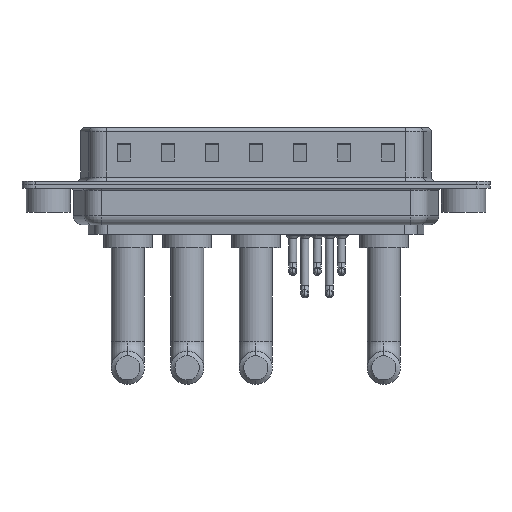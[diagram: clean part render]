
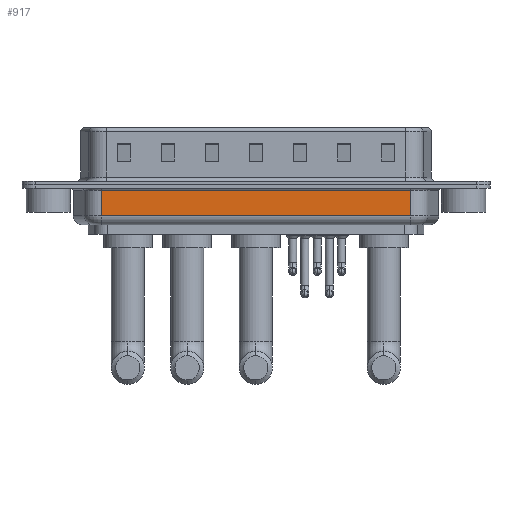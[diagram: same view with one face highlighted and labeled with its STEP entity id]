
A CAD part, front view. The second image highlights one B-rep face of the part: STEP entity #917.
In plain terms, the highlighted planar face has unit normal (0, -1, 0).
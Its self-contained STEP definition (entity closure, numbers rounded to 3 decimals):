
#821 = LINE ( 'NONE', #9465, #14283 ) ;
#917 = ADVANCED_FACE ( 'NONE', ( #13950 ), #20896, .F. ) ;
#1892 = DIRECTION ( 'NONE',  ( 0., 1., 0. ) ) ;
#2597 = CARTESIAN_POINT ( 'NONE',  ( 41.044, -5.35, -0.65 ) ) ;
#3189 = CARTESIAN_POINT ( 'NONE',  ( 6.006, -5.35, -0.65 ) ) ;
#3384 = EDGE_CURVE ( 'NONE', #19903, #16045, #821, .T. ) ;
#3623 = CARTESIAN_POINT ( 'NONE',  ( 6.006, -5.35, -0.65 ) ) ;
#4124 = DIRECTION ( 'NONE',  ( 1., 0., 0. ) ) ;
#4196 = EDGE_LOOP ( 'NONE', ( #12258, #13780, #5738, #14196 ) ) ;
#4897 = LINE ( 'NONE', #3189, #21410 ) ;
#5312 = CARTESIAN_POINT ( 'NONE',  ( 6.006, -5.35, -4.5 ) ) ;
#5525 = AXIS2_PLACEMENT_3D ( 'NONE', #5312, #1892, #8825 ) ;
#5738 = ORIENTED_EDGE ( 'NONE', *, *, #10011, .T. ) ;
#6715 = DIRECTION ( 'NONE',  ( 0., 0., 1. ) ) ;
#7554 = LINE ( 'NONE', #18985, #12543 ) ;
#8825 = DIRECTION ( 'NONE',  ( 0., 0., 1. ) ) ;
#9400 = VECTOR ( 'NONE', #6715, 1000. ) ;
#9465 = CARTESIAN_POINT ( 'NONE',  ( 6.006, -5.35, -3.5 ) ) ;
#10011 = EDGE_CURVE ( 'NONE', #16045, #12771, #7554, .T. ) ;
#12258 = ORIENTED_EDGE ( 'NONE', *, *, #15042, .F. ) ;
#12543 = VECTOR ( 'NONE', #22399, 1000. ) ;
#12771 = VERTEX_POINT ( 'NONE', #2597 ) ;
#12786 = LINE ( 'NONE', #19744, #9400 ) ;
#13290 = CARTESIAN_POINT ( 'NONE',  ( 6.006, -5.35, -3.5 ) ) ;
#13780 = ORIENTED_EDGE ( 'NONE', *, *, #3384, .T. ) ;
#13950 = FACE_OUTER_BOUND ( 'NONE', #4196, .T. ) ;
#14196 = ORIENTED_EDGE ( 'NONE', *, *, #15133, .T. ) ;
#14283 = VECTOR ( 'NONE', #4124, 1000. ) ;
#15042 = EDGE_CURVE ( 'NONE', #19903, #15296, #12786, .T. ) ;
#15133 = EDGE_CURVE ( 'NONE', #12771, #15296, #4897, .T. ) ;
#15296 = VERTEX_POINT ( 'NONE', #3623 ) ;
#16045 = VERTEX_POINT ( 'NONE', #19720 ) ;
#18985 = CARTESIAN_POINT ( 'NONE',  ( 41.044, -5.35, -4.5 ) ) ;
#19720 = CARTESIAN_POINT ( 'NONE',  ( 41.044, -5.35, -3.5 ) ) ;
#19744 = CARTESIAN_POINT ( 'NONE',  ( 6.006, -5.35, -4.5 ) ) ;
#19903 = VERTEX_POINT ( 'NONE', #13290 ) ;
#20896 = PLANE ( 'NONE',  #5525 ) ;
#21410 = VECTOR ( 'NONE', #22410, 1000. ) ;
#22399 = DIRECTION ( 'NONE',  ( 0., 0., 1. ) ) ;
#22410 = DIRECTION ( 'NONE',  ( -1., 0., 0. ) ) ;
